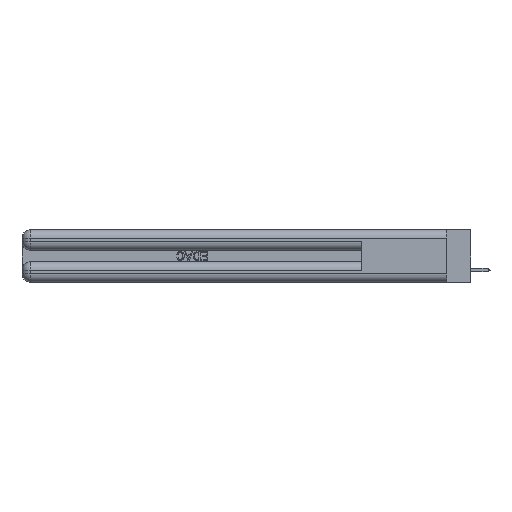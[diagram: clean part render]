
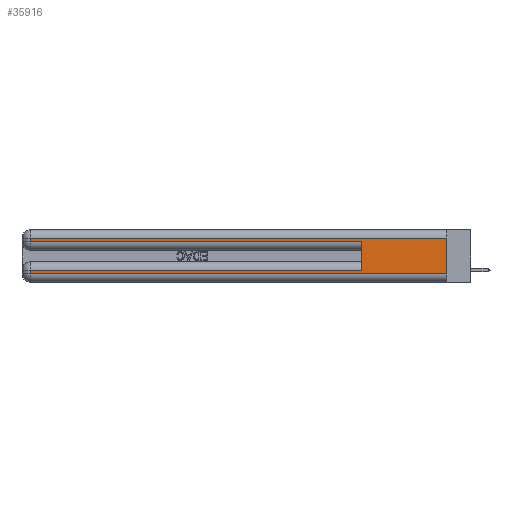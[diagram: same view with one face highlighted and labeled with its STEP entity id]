
A CAD part, left-side view. The second image highlights one B-rep face of the part: STEP entity #35916.
In plain terms, the highlighted planar face has unit normal (-1, 0, 0).
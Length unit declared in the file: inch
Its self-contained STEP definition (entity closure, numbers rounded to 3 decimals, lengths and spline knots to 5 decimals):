
#1373 = EDGE_CURVE ( 'NONE', #15557, #11618, #25684, .T. ) ;
#2459 = DIRECTION ( 'NONE',  ( 1., 0., 0. ) ) ;
#2921 = VERTEX_POINT ( 'NONE', #34415 ) ;
#3943 = VERTEX_POINT ( 'NONE', #21966 ) ;
#4300 = LINE ( 'NONE', #29617, #8915 ) ;
#5154 = VECTOR ( 'NONE', #23759, 39.37008 ) ;
#7550 = CARTESIAN_POINT ( 'NONE',  ( 0., 0., 0.31 ) ) ;
#8851 = VERTEX_POINT ( 'NONE', #24217 ) ;
#8915 = VECTOR ( 'NONE', #40604, 39.37008 ) ;
#10521 = DIRECTION ( 'NONE',  ( 0., 0., -1. ) ) ;
#10972 = EDGE_CURVE ( 'NONE', #2921, #32753, #15616, .T. ) ;
#11351 = DIRECTION ( 'NONE',  ( 0., 0., 1. ) ) ;
#11564 = ORIENTED_EDGE ( 'NONE', *, *, #10972, .T. ) ;
#11618 = VERTEX_POINT ( 'NONE', #42893 ) ;
#12515 = VECTOR ( 'NONE', #29691, 39.37008 ) ;
#13700 = PLANE ( 'NONE',  #17411 ) ;
#14000 = CARTESIAN_POINT ( 'NONE',  ( 0., 0., 0.285 ) ) ;
#14817 = DIRECTION ( 'NONE',  ( 0., -1., 0. ) ) ;
#14877 = CARTESIAN_POINT ( 'NONE',  ( 0., 0.6, 0.145 ) ) ;
#15169 = CARTESIAN_POINT ( 'NONE',  ( 0., 2.94, 0.06 ) ) ;
#15557 = VERTEX_POINT ( 'NONE', #38925 ) ;
#15616 = LINE ( 'NONE', #29600, #17870 ) ;
#16053 = CARTESIAN_POINT ( 'NONE',  ( 0., 0., 0.06 ) ) ;
#17411 = AXIS2_PLACEMENT_3D ( 'NONE', #32127, #2459, #28148 ) ;
#17741 = ORIENTED_EDGE ( 'NONE', *, *, #44357, .T. ) ;
#17870 = VECTOR ( 'NONE', #10521, 39.37008 ) ;
#20144 = CARTESIAN_POINT ( 'NONE',  ( 0., 2.94, 0.285 ) ) ;
#20429 = ORIENTED_EDGE ( 'NONE', *, *, #1373, .T. ) ;
#21966 = CARTESIAN_POINT ( 'NONE',  ( 0., 0.6, 0.285 ) ) ;
#22277 = LINE ( 'NONE', #37747, #45127 ) ;
#22893 = EDGE_LOOP ( 'NONE', ( #30893, #20429, #26655, #42748, #29271, #17741, #11564, #24401 ) ) ;
#23759 = DIRECTION ( 'NONE',  ( 0., -1., 0. ) ) ;
#24217 = CARTESIAN_POINT ( 'NONE',  ( 0., 0.6, 0.085 ) ) ;
#24401 = ORIENTED_EDGE ( 'NONE', *, *, #38729, .T. ) ;
#25684 = LINE ( 'NONE', #7550, #12515 ) ;
#26655 = ORIENTED_EDGE ( 'NONE', *, *, #28232, .T. ) ;
#27700 = VERTEX_POINT ( 'NONE', #36568 ) ;
#28089 = VECTOR ( 'NONE', #14817, 39.37008 ) ;
#28148 = DIRECTION ( 'NONE',  ( 0., 0., -1. ) ) ;
#28232 = EDGE_CURVE ( 'NONE', #11618, #29136, #44453, .T. ) ;
#28719 = CARTESIAN_POINT ( 'NONE',  ( 0., 2.94, 0.37 ) ) ;
#29136 = VERTEX_POINT ( 'NONE', #20144 ) ;
#29271 = ORIENTED_EDGE ( 'NONE', *, *, #44363, .F. ) ;
#29600 = CARTESIAN_POINT ( 'NONE',  ( 0., 2.94, 0.37 ) ) ;
#29617 = CARTESIAN_POINT ( 'NONE',  ( 0., 0., 0.085 ) ) ;
#29691 = DIRECTION ( 'NONE',  ( 0., 1., 0. ) ) ;
#30094 = DIRECTION ( 'NONE',  ( 0., 0., -1. ) ) ;
#30893 = ORIENTED_EDGE ( 'NONE', *, *, #34430, .F. ) ;
#32127 = CARTESIAN_POINT ( 'NONE',  ( 0., 0., 0.37 ) ) ;
#32396 = DIRECTION ( 'NONE',  ( 0., 0., -1. ) ) ;
#32402 = VECTOR ( 'NONE', #11351, 39.37008 ) ;
#32753 = VERTEX_POINT ( 'NONE', #15169 ) ;
#34415 = CARTESIAN_POINT ( 'NONE',  ( 0., 2.94, 0.085 ) ) ;
#34430 = EDGE_CURVE ( 'NONE', #15557, #27700, #22277, .T. ) ;
#35916 = ADVANCED_FACE ( 'NONE', ( #43140 ), #13700, .F. ) ;
#36013 = LINE ( 'NONE', #14000, #28089 ) ;
#36568 = CARTESIAN_POINT ( 'NONE',  ( 0., 0., 0.06 ) ) ;
#37747 = CARTESIAN_POINT ( 'NONE',  ( 0., 0., 0.37 ) ) ;
#38729 = EDGE_CURVE ( 'NONE', #32753, #27700, #44022, .T. ) ;
#38925 = CARTESIAN_POINT ( 'NONE',  ( 0., 0., 0.31 ) ) ;
#40604 = DIRECTION ( 'NONE',  ( 0., 1., 0. ) ) ;
#42092 = LINE ( 'NONE', #14877, #32402 ) ;
#42748 = ORIENTED_EDGE ( 'NONE', *, *, #47008, .T. ) ;
#42893 = CARTESIAN_POINT ( 'NONE',  ( 0., 2.94, 0.31 ) ) ;
#43140 = FACE_OUTER_BOUND ( 'NONE', #22893, .T. ) ;
#44022 = LINE ( 'NONE', #16053, #5154 ) ;
#44357 = EDGE_CURVE ( 'NONE', #8851, #2921, #4300, .T. ) ;
#44363 = EDGE_CURVE ( 'NONE', #8851, #3943, #42092, .T. ) ;
#44453 = LINE ( 'NONE', #28719, #45617 ) ;
#45127 = VECTOR ( 'NONE', #30094, 39.37008 ) ;
#45617 = VECTOR ( 'NONE', #32396, 39.37008 ) ;
#47008 = EDGE_CURVE ( 'NONE', #29136, #3943, #36013, .T. ) ;
